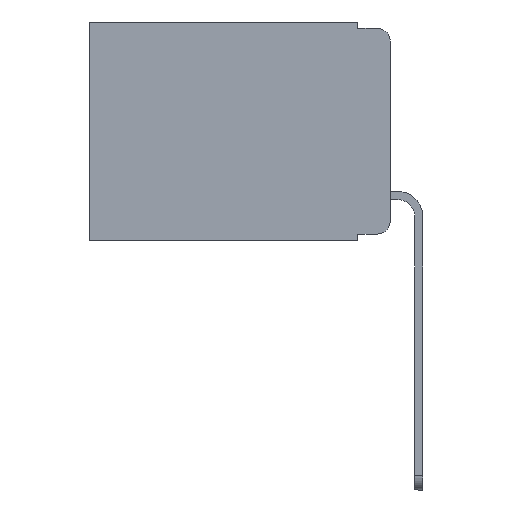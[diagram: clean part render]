
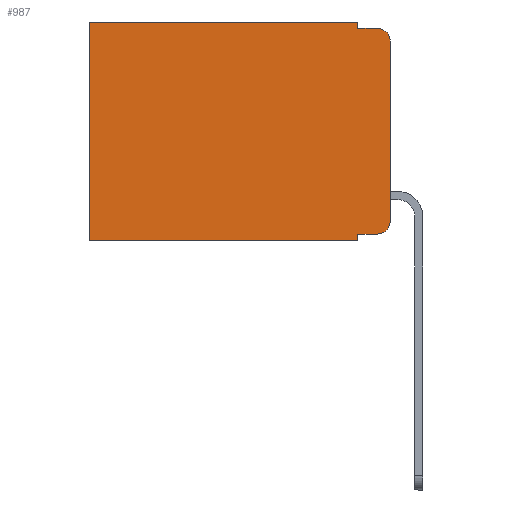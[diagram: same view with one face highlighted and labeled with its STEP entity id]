
A CAD part, left-side view. The second image highlights one B-rep face of the part: STEP entity #987.
In plain terms, the highlighted planar face has unit normal (-1, 0, 0).
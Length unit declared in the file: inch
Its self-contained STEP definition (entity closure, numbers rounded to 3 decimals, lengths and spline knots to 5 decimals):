
#160 = DIRECTION ( 'NONE',  ( 0., -1., 0. ) ) ;
#484 = ORIENTED_EDGE ( 'NONE', *, *, #8091, .T. ) ;
#510 = CARTESIAN_POINT ( 'NONE',  ( 0.298, 0.02, -0.333 ) ) ;
#570 = CARTESIAN_POINT ( 'NONE',  ( 0.298, 0.051, -0.343 ) ) ;
#767 = CARTESIAN_POINT ( 'NONE',  ( 0.298, 0., -0.313 ) ) ;
#772 = CARTESIAN_POINT ( 'NONE',  ( 0.298, 0.473, 0. ) ) ;
#987 = ADVANCED_FACE ( 'NONE', ( #2524 ), #7020, .F. ) ;
#1081 = ORIENTED_EDGE ( 'NONE', *, *, #5773, .T. ) ;
#1104 = VERTEX_POINT ( 'NONE', #5565 ) ;
#1230 = DIRECTION ( 'NONE',  ( 0., 0., -1. ) ) ;
#1271 = CARTESIAN_POINT ( 'NONE',  ( 0.298, 0., 0. ) ) ;
#1322 = LINE ( 'NONE', #6780, #8697 ) ;
#1342 = CARTESIAN_POINT ( 'NONE',  ( 0.298, 0.051, -0.333 ) ) ;
#1467 = VERTEX_POINT ( 'NONE', #767 ) ;
#1490 = LINE ( 'NONE', #12701, #11302 ) ;
#1705 = EDGE_CURVE ( 'NONE', #3933, #1104, #1490, .T. ) ;
#1930 = DIRECTION ( 'NONE',  ( 0., 0., -1. ) ) ;
#2200 = CARTESIAN_POINT ( 'NONE',  ( 0.298, 0.02, -0.313 ) ) ;
#2524 = FACE_OUTER_BOUND ( 'NONE', #11218, .T. ) ;
#2577 = DIRECTION ( 'NONE',  ( 0., 0., -1. ) ) ;
#2846 = ORIENTED_EDGE ( 'NONE', *, *, #12347, .T. ) ;
#2890 = CARTESIAN_POINT ( 'NONE',  ( 0.298, 0.02, -0.03 ) ) ;
#3010 = VERTEX_POINT ( 'NONE', #13875 ) ;
#3059 = DIRECTION ( 'NONE',  ( 0., 0., -1. ) ) ;
#3315 = DIRECTION ( 'NONE',  ( -1., 0., 0. ) ) ;
#3359 = VERTEX_POINT ( 'NONE', #11580 ) ;
#3933 = VERTEX_POINT ( 'NONE', #570 ) ;
#3961 = LINE ( 'NONE', #7132, #9824 ) ;
#4097 = LINE ( 'NONE', #772, #9726 ) ;
#4119 = CARTESIAN_POINT ( 'NONE',  ( 0.298, 0.473, 0. ) ) ;
#4441 = VERTEX_POINT ( 'NONE', #14458 ) ;
#4656 = DIRECTION ( 'NONE',  ( 0., 0., -1. ) ) ;
#5142 = DIRECTION ( 'NONE',  ( 0., 1., 0. ) ) ;
#5156 = VECTOR ( 'NONE', #3059, 39.37008 ) ;
#5286 = VERTEX_POINT ( 'NONE', #4119 ) ;
#5565 = CARTESIAN_POINT ( 'NONE',  ( 0.298, 0.473, -0.343 ) ) ;
#5694 = DIRECTION ( 'NONE',  ( 1., 0., 0. ) ) ;
#5773 = EDGE_CURVE ( 'NONE', #14566, #13169, #12548, .T. ) ;
#5794 = CARTESIAN_POINT ( 'NONE',  ( 0.298, 0., -0.03 ) ) ;
#6097 = EDGE_CURVE ( 'NONE', #14566, #3933, #13348, .T. ) ;
#6156 = DIRECTION ( 'NONE',  ( 0., 0., -1. ) ) ;
#6468 = VECTOR ( 'NONE', #1930, 39.37008 ) ;
#6665 = EDGE_CURVE ( 'NONE', #13169, #1467, #9891, .T. ) ;
#6780 = CARTESIAN_POINT ( 'NONE',  ( 0.298, 0.051, 0. ) ) ;
#6847 = EDGE_CURVE ( 'NONE', #10907, #1467, #8661, .T. ) ;
#7020 = PLANE ( 'NONE',  #9491 ) ;
#7096 = DIRECTION ( 'NONE',  ( 0., 1., 0. ) ) ;
#7132 = CARTESIAN_POINT ( 'NONE',  ( 0.298, 0., 0. ) ) ;
#7165 = DIRECTION ( 'NONE',  ( -1., 0., 0. ) ) ;
#7571 = EDGE_CURVE ( 'NONE', #4441, #3010, #1322, .T. ) ;
#7745 = CARTESIAN_POINT ( 'NONE',  ( 0.298, 0.051, 0. ) ) ;
#7969 = ORIENTED_EDGE ( 'NONE', *, *, #6097, .F. ) ;
#8086 = EDGE_CURVE ( 'NONE', #3010, #3359, #10587, .T. ) ;
#8091 = EDGE_CURVE ( 'NONE', #4441, #5286, #3961, .T. ) ;
#8582 = VECTOR ( 'NONE', #160, 39.37008 ) ;
#8660 = AXIS2_PLACEMENT_3D ( 'NONE', #2890, #7165, #10552 ) ;
#8661 = LINE ( 'NONE', #13087, #5156 ) ;
#8697 = VECTOR ( 'NONE', #2577, 39.37008 ) ;
#9307 = ORIENTED_EDGE ( 'NONE', *, *, #8086, .F. ) ;
#9491 = AXIS2_PLACEMENT_3D ( 'NONE', #1271, #5694, #4656 ) ;
#9492 = ORIENTED_EDGE ( 'NONE', *, *, #1705, .F. ) ;
#9726 = VECTOR ( 'NONE', #6156, 39.37008 ) ;
#9824 = VECTOR ( 'NONE', #5142, 39.37008 ) ;
#9891 = CIRCLE ( 'NONE', #12723, 0.02 ) ;
#10552 = DIRECTION ( 'NONE',  ( 0., 0., -1. ) ) ;
#10587 = LINE ( 'NONE', #10657, #12408 ) ;
#10657 = CARTESIAN_POINT ( 'NONE',  ( 0.298, 0.051, -0.01 ) ) ;
#10860 = ORIENTED_EDGE ( 'NONE', *, *, #6847, .F. ) ;
#10907 = VERTEX_POINT ( 'NONE', #5794 ) ;
#11218 = EDGE_LOOP ( 'NONE', ( #10860, #13676, #9307, #11840, #484, #2846, #9492, #7969, #1081, #11735 ) ) ;
#11302 = VECTOR ( 'NONE', #7096, 39.37008 ) ;
#11533 = EDGE_CURVE ( 'NONE', #10907, #3359, #11714, .T. ) ;
#11580 = CARTESIAN_POINT ( 'NONE',  ( 0.298, 0.02, -0.01 ) ) ;
#11714 = CIRCLE ( 'NONE', #8660, 0.02 ) ;
#11735 = ORIENTED_EDGE ( 'NONE', *, *, #6665, .T. ) ;
#11840 = ORIENTED_EDGE ( 'NONE', *, *, #7571, .F. ) ;
#12347 = EDGE_CURVE ( 'NONE', #5286, #1104, #4097, .T. ) ;
#12354 = CARTESIAN_POINT ( 'NONE',  ( 0.298, 0.051, -0.333 ) ) ;
#12408 = VECTOR ( 'NONE', #14133, 39.37008 ) ;
#12548 = LINE ( 'NONE', #1342, #8582 ) ;
#12701 = CARTESIAN_POINT ( 'NONE',  ( 0.298, 0., -0.343 ) ) ;
#12723 = AXIS2_PLACEMENT_3D ( 'NONE', #2200, #3315, #1230 ) ;
#13087 = CARTESIAN_POINT ( 'NONE',  ( 0.298, 0., 0. ) ) ;
#13169 = VERTEX_POINT ( 'NONE', #510 ) ;
#13348 = LINE ( 'NONE', #7745, #6468 ) ;
#13676 = ORIENTED_EDGE ( 'NONE', *, *, #11533, .T. ) ;
#13875 = CARTESIAN_POINT ( 'NONE',  ( 0.298, 0.051, -0.01 ) ) ;
#14133 = DIRECTION ( 'NONE',  ( 0., -1., 0. ) ) ;
#14458 = CARTESIAN_POINT ( 'NONE',  ( 0.298, 0.051, 0. ) ) ;
#14566 = VERTEX_POINT ( 'NONE', #12354 ) ;
